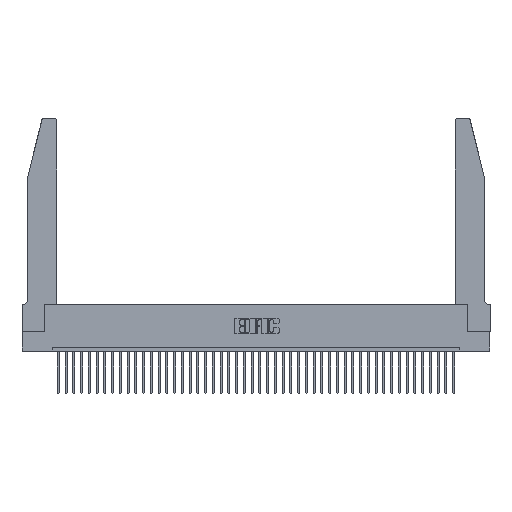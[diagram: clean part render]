
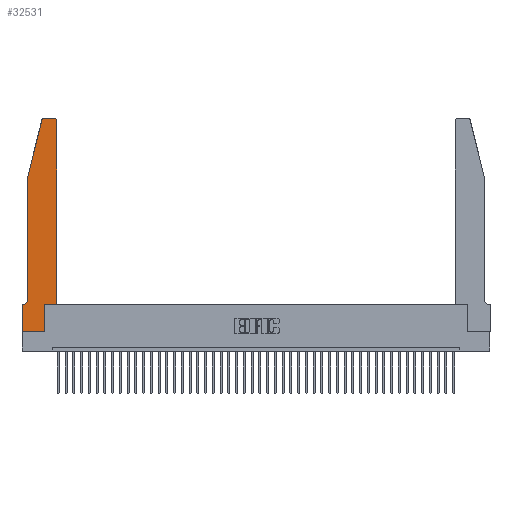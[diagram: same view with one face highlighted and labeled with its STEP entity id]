
A CAD part, top view. The second image highlights one B-rep face of the part: STEP entity #32531.
In plain terms, the highlighted planar face has unit normal (0, 0, 1).
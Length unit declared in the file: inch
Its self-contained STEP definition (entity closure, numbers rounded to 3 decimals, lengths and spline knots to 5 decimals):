
#305 = VERTEX_POINT ( 'NONE', #10868 ) ;
#728 = VERTEX_POINT ( 'NONE', #25791 ) ;
#1252 = LINE ( 'NONE', #13255, #2300 ) ;
#1348 = DIRECTION ( 'NONE',  ( -1., 0., 0. ) ) ;
#1816 = VERTEX_POINT ( 'NONE', #15280 ) ;
#2178 = VERTEX_POINT ( 'NONE', #8558 ) ;
#2300 = VECTOR ( 'NONE', #42568, 39.37008 ) ;
#2563 = CARTESIAN_POINT ( 'NONE',  ( 0.2605, 2.75, 0.37 ) ) ;
#2811 = ORIENTED_EDGE ( 'NONE', *, *, #33864, .T. ) ;
#3593 = LINE ( 'NONE', #37225, #27704 ) ;
#3887 = CARTESIAN_POINT ( 'NONE',  ( 0., 0.35, 0.37 ) ) ;
#4170 = CARTESIAN_POINT ( 'NONE',  ( 0., 0., 0.37 ) ) ;
#4281 = EDGE_CURVE ( 'NONE', #20842, #5919, #27908, .T. ) ;
#4805 = CARTESIAN_POINT ( 'NONE',  ( 0.4205, 2.75, 0.37 ) ) ;
#5092 = EDGE_CURVE ( 'NONE', #25879, #1816, #24302, .T. ) ;
#5919 = VERTEX_POINT ( 'NONE', #13464 ) ;
#6257 = DIRECTION ( 'NONE',  ( -1., 0., 0. ) ) ;
#7553 = AXIS2_PLACEMENT_3D ( 'NONE', #29898, #20132, #13549 ) ;
#7993 = CARTESIAN_POINT ( 'NONE',  ( 0.2865, 0.35, 0.37 ) ) ;
#8252 = VECTOR ( 'NONE', #41724, 39.37008 ) ;
#8558 = CARTESIAN_POINT ( 'NONE',  ( 0.25487, 2.72718, 0.37 ) ) ;
#10868 = CARTESIAN_POINT ( 'NONE',  ( 0.4505, 0.35, 0.37 ) ) ;
#10893 = CARTESIAN_POINT ( 'NONE',  ( 0., 0.35, 0.37 ) ) ;
#11064 = LINE ( 'NONE', #31587, #41413 ) ;
#11185 = DIRECTION ( 'NONE',  ( 1., 0., 0. ) ) ;
#11237 = EDGE_CURVE ( 'NONE', #305, #728, #1252, .T. ) ;
#11411 = DIRECTION ( 'NONE',  ( 1., 0., 0. ) ) ;
#12366 = ORIENTED_EDGE ( 'NONE', *, *, #32543, .T. ) ;
#12628 = CARTESIAN_POINT ( 'NONE',  ( 0.0055, 0.35, 0.37 ) ) ;
#13255 = CARTESIAN_POINT ( 'NONE',  ( 0.4505, 0.35, 0.37 ) ) ;
#13464 = CARTESIAN_POINT ( 'NONE',  ( 0.284, 2.75, 0.37 ) ) ;
#13549 = DIRECTION ( 'NONE',  ( 1., 0., 0. ) ) ;
#15236 = AXIS2_PLACEMENT_3D ( 'NONE', #31077, #20746, #11411 ) ;
#15280 = CARTESIAN_POINT ( 'NONE',  ( 0.2865, 0., 0.37 ) ) ;
#15390 = CARTESIAN_POINT ( 'NONE',  ( 0.0755, 2., 0.37 ) ) ;
#16601 = PLANE ( 'NONE',  #33447 ) ;
#16853 = ORIENTED_EDGE ( 'NONE', *, *, #39619, .T. ) ;
#16998 = FACE_OUTER_BOUND ( 'NONE', #27540, .T. ) ;
#17426 = EDGE_CURVE ( 'NONE', #21972, #305, #42338, .T. ) ;
#18515 = CARTESIAN_POINT ( 'NONE',  ( 0.0755, 2., 0.37 ) ) ;
#18785 = EDGE_CURVE ( 'NONE', #5919, #2178, #19070, .T. ) ;
#19070 = CIRCLE ( 'NONE', #7553, 0.03 ) ;
#19778 = VECTOR ( 'NONE', #24669, 39.37008 ) ;
#19855 = CIRCLE ( 'NONE', #27503, 0.07 ) ;
#20132 = DIRECTION ( 'NONE',  ( 0., 0., 1. ) ) ;
#20321 = EDGE_CURVE ( 'NONE', #728, #20842, #23623, .T. ) ;
#20746 = DIRECTION ( 'NONE',  ( 0., 0., 1. ) ) ;
#20823 = LINE ( 'NONE', #34596, #19778 ) ;
#20842 = VERTEX_POINT ( 'NONE', #4805 ) ;
#20912 = DIRECTION ( 'NONE',  ( 0., -1., 0. ) ) ;
#21280 = ORIENTED_EDGE ( 'NONE', *, *, #17426, .T. ) ;
#21972 = VERTEX_POINT ( 'NONE', #7993 ) ;
#22077 = LINE ( 'NONE', #15390, #8252 ) ;
#22213 = VECTOR ( 'NONE', #29283, 39.37008 ) ;
#22793 = EDGE_CURVE ( 'NONE', #1816, #21972, #11064, .T. ) ;
#23530 = DIRECTION ( 'NONE',  ( 1., 0., 0. ) ) ;
#23623 = CIRCLE ( 'NONE', #15236, 0.03 ) ;
#24267 = CARTESIAN_POINT ( 'NONE',  ( 0.4505, 0.35, 0.37 ) ) ;
#24302 = LINE ( 'NONE', #35921, #22213 ) ;
#24669 = DIRECTION ( 'NONE',  ( -0.239, -0.971, 0. ) ) ;
#24827 = VECTOR ( 'NONE', #28081, 39.37008 ) ;
#25116 = CARTESIAN_POINT ( 'NONE',  ( 0.0755, 0.42, 0.37 ) ) ;
#25285 = LINE ( 'NONE', #4170, #40674 ) ;
#25791 = CARTESIAN_POINT ( 'NONE',  ( 0.4505, 2.72, 0.37 ) ) ;
#25879 = VERTEX_POINT ( 'NONE', #28054 ) ;
#26118 = ORIENTED_EDGE ( 'NONE', *, *, #11237, .T. ) ;
#27047 = VERTEX_POINT ( 'NONE', #25116 ) ;
#27503 = AXIS2_PLACEMENT_3D ( 'NONE', #42294, #32358, #6257 ) ;
#27540 = EDGE_LOOP ( 'NONE', ( #42144, #38291, #28185, #41731, #16853, #2811, #12366, #36963, #31938, #21280, #26118, #32972 ) ) ;
#27704 = VECTOR ( 'NONE', #1348, 39.37008 ) ;
#27908 = LINE ( 'NONE', #2563, #24827 ) ;
#28054 = CARTESIAN_POINT ( 'NONE',  ( 0., 0., 0.37 ) ) ;
#28081 = DIRECTION ( 'NONE',  ( -1., 0., 0. ) ) ;
#28185 = ORIENTED_EDGE ( 'NONE', *, *, #41771, .T. ) ;
#28662 = VERTEX_POINT ( 'NONE', #10893 ) ;
#29283 = DIRECTION ( 'NONE',  ( 1., 0., 0. ) ) ;
#29898 = CARTESIAN_POINT ( 'NONE',  ( 0.284, 2.72, 0.37 ) ) ;
#31013 = VECTOR ( 'NONE', #11185, 39.37008 ) ;
#31077 = CARTESIAN_POINT ( 'NONE',  ( 0.4205, 2.72, 0.37 ) ) ;
#31534 = VERTEX_POINT ( 'NONE', #18515 ) ;
#31587 = CARTESIAN_POINT ( 'NONE',  ( 0.2865, 0.35, 0.37 ) ) ;
#31938 = ORIENTED_EDGE ( 'NONE', *, *, #22793, .T. ) ;
#32358 = DIRECTION ( 'NONE',  ( 0., 0., -1. ) ) ;
#32531 = ADVANCED_FACE ( 'NONE', ( #16998 ), #16601, .T. ) ;
#32543 = EDGE_CURVE ( 'NONE', #28662, #25879, #25285, .T. ) ;
#32972 = ORIENTED_EDGE ( 'NONE', *, *, #20321, .T. ) ;
#33430 = EDGE_CURVE ( 'NONE', #31534, #27047, #22077, .T. ) ;
#33447 = AXIS2_PLACEMENT_3D ( 'NONE', #3887, #36873, #23530 ) ;
#33864 = EDGE_CURVE ( 'NONE', #34045, #28662, #3593, .T. ) ;
#34045 = VERTEX_POINT ( 'NONE', #12628 ) ;
#34596 = CARTESIAN_POINT ( 'NONE',  ( 0.0755, 2., 0.37 ) ) ;
#35921 = CARTESIAN_POINT ( 'NONE',  ( 0., 0., 0.37 ) ) ;
#36873 = DIRECTION ( 'NONE',  ( 0., 0., 1. ) ) ;
#36963 = ORIENTED_EDGE ( 'NONE', *, *, #5092, .T. ) ;
#37225 = CARTESIAN_POINT ( 'NONE',  ( 0.0755, 0.35, 0.37 ) ) ;
#38291 = ORIENTED_EDGE ( 'NONE', *, *, #18785, .T. ) ;
#39619 = EDGE_CURVE ( 'NONE', #27047, #34045, #19855, .T. ) ;
#40674 = VECTOR ( 'NONE', #20912, 39.37008 ) ;
#41413 = VECTOR ( 'NONE', #41529, 39.37008 ) ;
#41529 = DIRECTION ( 'NONE',  ( 0., 1., 0. ) ) ;
#41724 = DIRECTION ( 'NONE',  ( 0., -1., 0. ) ) ;
#41731 = ORIENTED_EDGE ( 'NONE', *, *, #33430, .T. ) ;
#41771 = EDGE_CURVE ( 'NONE', #2178, #31534, #20823, .T. ) ;
#42144 = ORIENTED_EDGE ( 'NONE', *, *, #4281, .T. ) ;
#42294 = CARTESIAN_POINT ( 'NONE',  ( 0.0055, 0.42, 0.37 ) ) ;
#42338 = LINE ( 'NONE', #24267, #31013 ) ;
#42568 = DIRECTION ( 'NONE',  ( 0., 1., 0. ) ) ;
